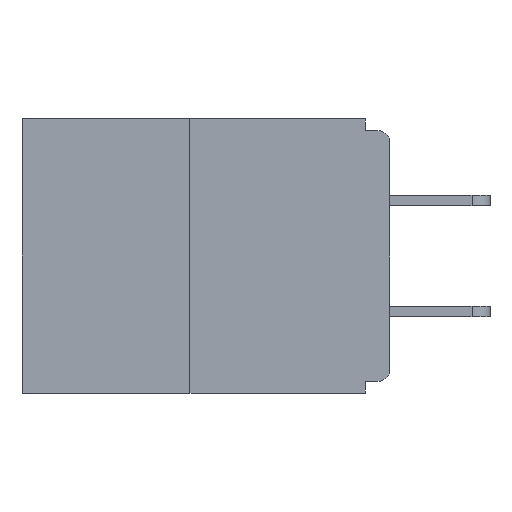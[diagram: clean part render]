
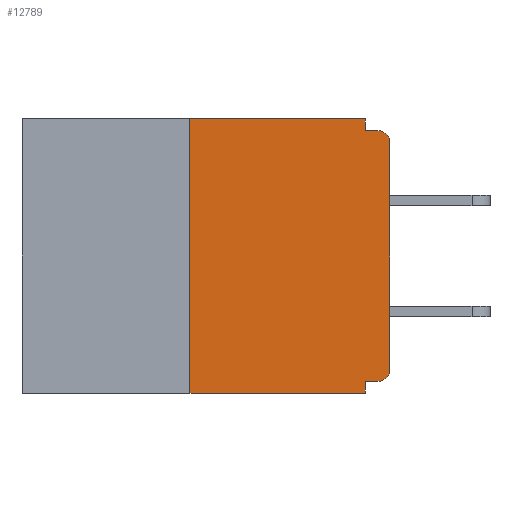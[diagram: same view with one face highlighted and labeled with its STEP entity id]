
A CAD part, left-side view. The second image highlights one B-rep face of the part: STEP entity #12789.
In plain terms, the highlighted planar face has unit normal (-1, 0, 0).
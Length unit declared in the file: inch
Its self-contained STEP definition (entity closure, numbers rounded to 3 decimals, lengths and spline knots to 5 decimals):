
#685 = VERTEX_POINT ( 'NONE', #16919 ) ;
#696 = ORIENTED_EDGE ( 'NONE', *, *, #18042, .F. ) ;
#870 = LINE ( 'NONE', #12222, #5322 ) ;
#1012 = DIRECTION ( 'NONE',  ( -1., 0., 0. ) ) ;
#1079 = DIRECTION ( 'NONE',  ( 0., 0., 1. ) ) ;
#1088 = CARTESIAN_POINT ( 'NONE',  ( 0., 0.015, -0.03 ) ) ;
#1366 = CARTESIAN_POINT ( 'NONE',  ( 0., 0.031, -0.015 ) ) ;
#1397 = DIRECTION ( 'NONE',  ( 0., 0., 1. ) ) ;
#1400 = EDGE_CURVE ( 'NONE', #1530, #11760, #5823, .T. ) ;
#1530 = VERTEX_POINT ( 'NONE', #7951 ) ;
#1622 = PLANE ( 'NONE',  #6266 ) ;
#1898 = ORIENTED_EDGE ( 'NONE', *, *, #8421, .F. ) ;
#2185 = ORIENTED_EDGE ( 'NONE', *, *, #5511, .T. ) ;
#2321 = CARTESIAN_POINT ( 'NONE',  ( 0., 0.031, -0.328 ) ) ;
#2784 = VECTOR ( 'NONE', #12125, 39.37008 ) ;
#2883 = DIRECTION ( 'NONE',  ( 0., 0., -1. ) ) ;
#3678 = VECTOR ( 'NONE', #17010, 39.37008 ) ;
#3850 = VECTOR ( 'NONE', #19910, 39.37008 ) ;
#3934 = VECTOR ( 'NONE', #1079, 39.37008 ) ;
#4100 = VERTEX_POINT ( 'NONE', #8409 ) ;
#4119 = ORIENTED_EDGE ( 'NONE', *, *, #8180, .F. ) ;
#4426 = VERTEX_POINT ( 'NONE', #16023 ) ;
#4685 = CARTESIAN_POINT ( 'NONE',  ( 0., 0., 0. ) ) ;
#5322 = VECTOR ( 'NONE', #5363, 39.37008 ) ;
#5363 = DIRECTION ( 'NONE',  ( 0., 1., 0. ) ) ;
#5511 = EDGE_CURVE ( 'NONE', #20357, #685, #15781, .T. ) ;
#5823 = LINE ( 'NONE', #8905, #3678 ) ;
#5932 = FACE_OUTER_BOUND ( 'NONE', #8354, .T. ) ;
#6113 = EDGE_CURVE ( 'NONE', #4426, #7654, #870, .T. ) ;
#6266 = AXIS2_PLACEMENT_3D ( 'NONE', #16597, #18194, #13230 ) ;
#6504 = VECTOR ( 'NONE', #1397, 39.37008 ) ;
#6522 = DIRECTION ( 'NONE',  ( 0., -1., 0. ) ) ;
#6558 = CARTESIAN_POINT ( 'NONE',  ( 0., 0.031, 0. ) ) ;
#6909 = CARTESIAN_POINT ( 'NONE',  ( 0., 0., -0.03 ) ) ;
#7014 = LINE ( 'NONE', #4685, #6504 ) ;
#7637 = VERTEX_POINT ( 'NONE', #18818 ) ;
#7654 = VERTEX_POINT ( 'NONE', #2321 ) ;
#7951 = CARTESIAN_POINT ( 'NONE',  ( 0., 0.25, 0. ) ) ;
#8180 = EDGE_CURVE ( 'NONE', #19559, #4100, #20116, .T. ) ;
#8273 = ORIENTED_EDGE ( 'NONE', *, *, #1400, .F. ) ;
#8354 = EDGE_LOOP ( 'NONE', ( #8273, #696, #2185, #18687, #14545, #12488, #19352, #13927, #4119, #1898 ) ) ;
#8409 = CARTESIAN_POINT ( 'NONE',  ( 0., 0.015, -0.015 ) ) ;
#8421 = EDGE_CURVE ( 'NONE', #11760, #19559, #9097, .T. ) ;
#8578 = DIRECTION ( 'NONE',  ( 0., 0., -1. ) ) ;
#8704 = CARTESIAN_POINT ( 'NONE',  ( 0., 0.015, -0.313 ) ) ;
#8818 = CARTESIAN_POINT ( 'NONE',  ( 0., 0.031, -0.343 ) ) ;
#8905 = CARTESIAN_POINT ( 'NONE',  ( 0., 0.46, 0. ) ) ;
#9045 = EDGE_CURVE ( 'NONE', #7637, #9566, #7014, .T. ) ;
#9097 = LINE ( 'NONE', #6558, #3850 ) ;
#9385 = CARTESIAN_POINT ( 'NONE',  ( 0., 0.25, 0. ) ) ;
#9566 = VERTEX_POINT ( 'NONE', #6909 ) ;
#10908 = LINE ( 'NONE', #8818, #2784 ) ;
#11090 = CIRCLE ( 'NONE', #19877, 0.015 ) ;
#11760 = VERTEX_POINT ( 'NONE', #13419 ) ;
#12125 = DIRECTION ( 'NONE',  ( 0., 0., -1. ) ) ;
#12222 = CARTESIAN_POINT ( 'NONE',  ( 0., 0., -0.328 ) ) ;
#12488 = ORIENTED_EDGE ( 'NONE', *, *, #12857, .T. ) ;
#12515 = VECTOR ( 'NONE', #6522, 39.37008 ) ;
#12522 = EDGE_CURVE ( 'NONE', #7654, #685, #10908, .T. ) ;
#12789 = ADVANCED_FACE ( 'NONE', ( #5932 ), #1622, .F. ) ;
#12857 = EDGE_CURVE ( 'NONE', #4426, #7637, #18191, .T. ) ;
#13230 = DIRECTION ( 'NONE',  ( 0., 0., -1. ) ) ;
#13419 = CARTESIAN_POINT ( 'NONE',  ( 0., 0.031, 0. ) ) ;
#13927 = ORIENTED_EDGE ( 'NONE', *, *, #16859, .T. ) ;
#13965 = VECTOR ( 'NONE', #14234, 39.37008 ) ;
#14234 = DIRECTION ( 'NONE',  ( 0., -1., 0. ) ) ;
#14545 = ORIENTED_EDGE ( 'NONE', *, *, #6113, .F. ) ;
#15463 = LINE ( 'NONE', #9385, #3934 ) ;
#15479 = CARTESIAN_POINT ( 'NONE',  ( 0., 0.46, -0.343 ) ) ;
#15560 = CARTESIAN_POINT ( 'NONE',  ( 0., 0.25, -0.343 ) ) ;
#15781 = LINE ( 'NONE', #15479, #13965 ) ;
#16023 = CARTESIAN_POINT ( 'NONE',  ( 0., 0.015, -0.328 ) ) ;
#16597 = CARTESIAN_POINT ( 'NONE',  ( 0., 0.46, 0. ) ) ;
#16859 = EDGE_CURVE ( 'NONE', #9566, #4100, #11090, .T. ) ;
#16919 = CARTESIAN_POINT ( 'NONE',  ( 0., 0.031, -0.343 ) ) ;
#17010 = DIRECTION ( 'NONE',  ( 0., -1., 0. ) ) ;
#17443 = AXIS2_PLACEMENT_3D ( 'NONE', #8704, #18558, #8578 ) ;
#18042 = EDGE_CURVE ( 'NONE', #20357, #1530, #15463, .T. ) ;
#18191 = CIRCLE ( 'NONE', #17443, 0.015 ) ;
#18194 = DIRECTION ( 'NONE',  ( 1., 0., 0. ) ) ;
#18558 = DIRECTION ( 'NONE',  ( -1., 0., 0. ) ) ;
#18687 = ORIENTED_EDGE ( 'NONE', *, *, #12522, .F. ) ;
#18818 = CARTESIAN_POINT ( 'NONE',  ( 0., 0., -0.313 ) ) ;
#19352 = ORIENTED_EDGE ( 'NONE', *, *, #9045, .T. ) ;
#19559 = VERTEX_POINT ( 'NONE', #1366 ) ;
#19799 = CARTESIAN_POINT ( 'NONE',  ( 0., 0., -0.015 ) ) ;
#19877 = AXIS2_PLACEMENT_3D ( 'NONE', #1088, #1012, #2883 ) ;
#19910 = DIRECTION ( 'NONE',  ( 0., 0., -1. ) ) ;
#20116 = LINE ( 'NONE', #19799, #12515 ) ;
#20357 = VERTEX_POINT ( 'NONE', #15560 ) ;
